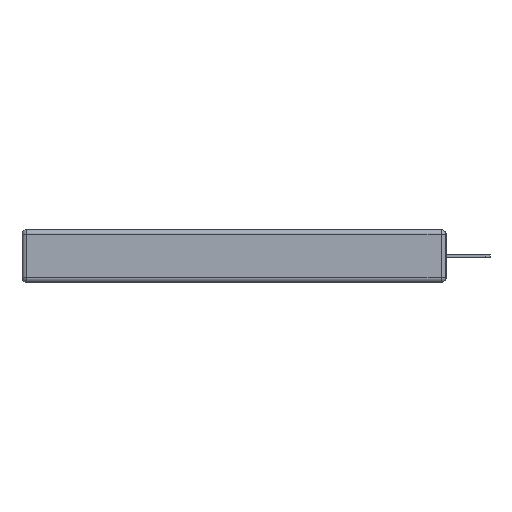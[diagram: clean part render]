
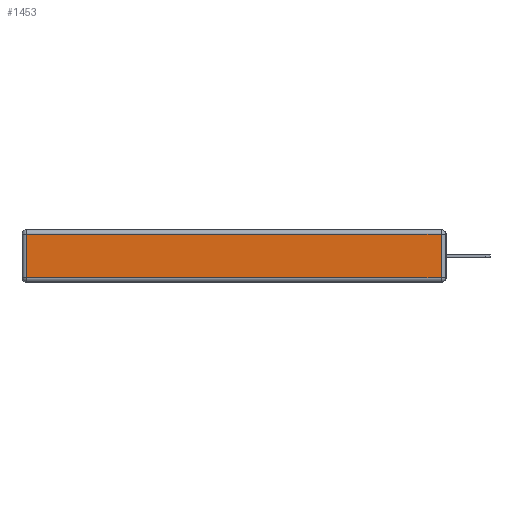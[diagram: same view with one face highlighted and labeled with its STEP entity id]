
A CAD part, left-side view. The second image highlights one B-rep face of the part: STEP entity #1453.
In plain terms, the highlighted planar face has unit normal (-1, 0, 0).
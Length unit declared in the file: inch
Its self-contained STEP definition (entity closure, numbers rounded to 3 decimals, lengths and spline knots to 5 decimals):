
#247 = DIRECTION ( 'NONE',  ( 0., 0., -1. ) ) ;
#1453 = ADVANCED_FACE ( 'NONE', ( #9591 ), #12018, .T. ) ;
#1636 = ORIENTED_EDGE ( 'NONE', *, *, #8939, .T. ) ;
#2977 = VECTOR ( 'NONE', #247, 39.37008 ) ;
#3210 = LINE ( 'NONE', #9293, #16079 ) ;
#3831 = VECTOR ( 'NONE', #4041, 39.37008 ) ;
#4041 = DIRECTION ( 'NONE',  ( 0., -1., 0. ) ) ;
#5466 = DIRECTION ( 'NONE',  ( 0., 0., 1. ) ) ;
#5977 = ORIENTED_EDGE ( 'NONE', *, *, #10096, .T. ) ;
#6092 = ORIENTED_EDGE ( 'NONE', *, *, #6355, .T. ) ;
#6355 = EDGE_CURVE ( 'NONE', #12584, #7544, #16226, .T. ) ;
#6559 = DIRECTION ( 'NONE',  ( 0., 1., 0. ) ) ;
#7544 = VERTEX_POINT ( 'NONE', #10420 ) ;
#7869 = EDGE_LOOP ( 'NONE', ( #5977, #1636, #9420, #6092 ) ) ;
#8130 = EDGE_CURVE ( 'NONE', #13305, #12584, #11421, .T. ) ;
#8385 = CARTESIAN_POINT ( 'NONE',  ( 0., 0.03, -0.313 ) ) ;
#8692 = CARTESIAN_POINT ( 'NONE',  ( 0., 0.03, -0.03 ) ) ;
#8939 = EDGE_CURVE ( 'NONE', #13131, #13305, #3210, .T. ) ;
#9149 = CARTESIAN_POINT ( 'NONE',  ( 0., 0., -0.313 ) ) ;
#9293 = CARTESIAN_POINT ( 'NONE',  ( 0., 0.03, -0.343 ) ) ;
#9420 = ORIENTED_EDGE ( 'NONE', *, *, #8130, .T. ) ;
#9591 = FACE_OUTER_BOUND ( 'NONE', #7869, .T. ) ;
#10096 = EDGE_CURVE ( 'NONE', #7544, #13131, #13422, .T. ) ;
#10420 = CARTESIAN_POINT ( 'NONE',  ( 0., 2.72, -0.313 ) ) ;
#10681 = CARTESIAN_POINT ( 'NONE',  ( 0., 2.72, -0.343 ) ) ;
#11421 = LINE ( 'NONE', #13987, #14604 ) ;
#11563 = DIRECTION ( 'NONE',  ( -1., 0., 0. ) ) ;
#11667 = CARTESIAN_POINT ( 'NONE',  ( 0., 0., -0.343 ) ) ;
#11802 = DIRECTION ( 'NONE',  ( 0., 0., 1. ) ) ;
#12018 = PLANE ( 'NONE',  #12365 ) ;
#12365 = AXIS2_PLACEMENT_3D ( 'NONE', #11667, #11563, #11802 ) ;
#12584 = VERTEX_POINT ( 'NONE', #15779 ) ;
#13131 = VERTEX_POINT ( 'NONE', #8385 ) ;
#13305 = VERTEX_POINT ( 'NONE', #8692 ) ;
#13422 = LINE ( 'NONE', #9149, #3831 ) ;
#13987 = CARTESIAN_POINT ( 'NONE',  ( 0., 2.75, -0.03 ) ) ;
#14604 = VECTOR ( 'NONE', #6559, 39.37008 ) ;
#15779 = CARTESIAN_POINT ( 'NONE',  ( 0., 2.72, -0.03 ) ) ;
#16079 = VECTOR ( 'NONE', #5466, 39.37008 ) ;
#16226 = LINE ( 'NONE', #10681, #2977 ) ;
